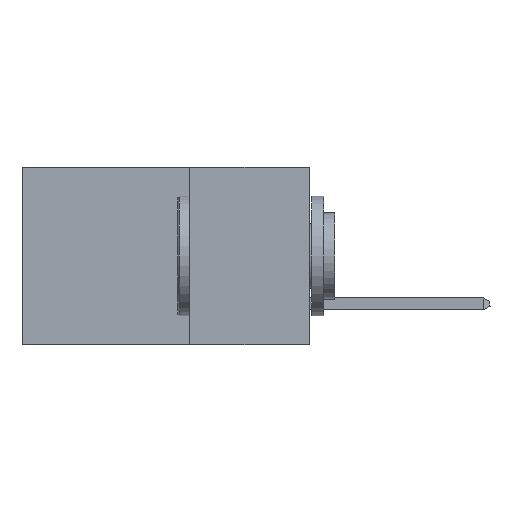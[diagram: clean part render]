
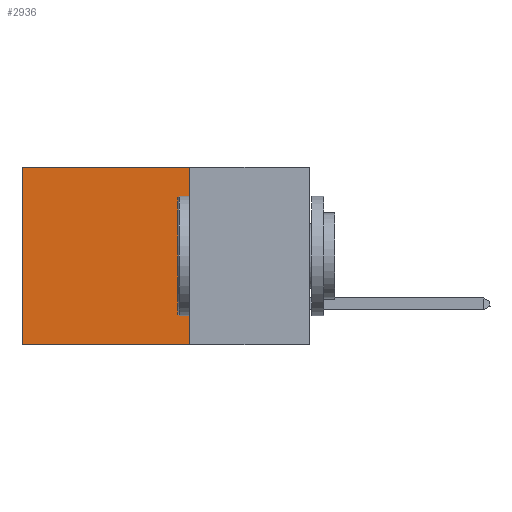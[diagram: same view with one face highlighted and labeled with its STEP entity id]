
A CAD part, left-side view. The second image highlights one B-rep face of the part: STEP entity #2936.
In plain terms, the highlighted planar face has unit normal (-1, 0, 0).
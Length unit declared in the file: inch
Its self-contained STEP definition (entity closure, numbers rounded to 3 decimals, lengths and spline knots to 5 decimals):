
#275 = VERTEX_POINT ( 'NONE', #2240 ) ;
#648 = VECTOR ( 'NONE', #9031, 39.37008 ) ;
#945 = EDGE_CURVE ( 'NONE', #275, #1674, #11428, .T. ) ;
#1343 = ORIENTED_EDGE ( 'NONE', *, *, #3459, .T. ) ;
#1512 = CARTESIAN_POINT ( 'NONE',  ( 0.2875, 0.6, 0. ) ) ;
#1674 = VERTEX_POINT ( 'NONE', #7368 ) ;
#2240 = CARTESIAN_POINT ( 'NONE',  ( 0.2875, 0.25, 0. ) ) ;
#2512 = DIRECTION ( 'NONE',  ( 1., 0., 0. ) ) ;
#2647 = AXIS2_PLACEMENT_3D ( 'NONE', #8001, #2512, #8926 ) ;
#2830 = CARTESIAN_POINT ( 'NONE',  ( 0.2875, 0.6, 0. ) ) ;
#2936 = ADVANCED_FACE ( 'NONE', ( #5419 ), #4305, .F. ) ;
#3459 = EDGE_CURVE ( 'NONE', #9494, #3676, #11874, .T. ) ;
#3676 = VERTEX_POINT ( 'NONE', #9169 ) ;
#3939 = DIRECTION ( 'NONE',  ( 0., 1., 0. ) ) ;
#4305 = PLANE ( 'NONE',  #2647 ) ;
#4887 = CARTESIAN_POINT ( 'NONE',  ( 0.2875, 0.25, 0. ) ) ;
#5370 = DIRECTION ( 'NONE',  ( 0., 0., -1. ) ) ;
#5419 = FACE_OUTER_BOUND ( 'NONE', #9442, .T. ) ;
#6614 = LINE ( 'NONE', #11047, #8190 ) ;
#7368 = CARTESIAN_POINT ( 'NONE',  ( 0.2875, 0.25, -0.37 ) ) ;
#8001 = CARTESIAN_POINT ( 'NONE',  ( 0.2875, 0.25, 0. ) ) ;
#8190 = VECTOR ( 'NONE', #3939, 39.37008 ) ;
#8768 = ORIENTED_EDGE ( 'NONE', *, *, #945, .F. ) ;
#8926 = DIRECTION ( 'NONE',  ( 0., 0., -1. ) ) ;
#9031 = DIRECTION ( 'NONE',  ( 0., 1., 0. ) ) ;
#9169 = CARTESIAN_POINT ( 'NONE',  ( 0.2875, 0.6, -0.37 ) ) ;
#9361 = ORIENTED_EDGE ( 'NONE', *, *, #11717, .T. ) ;
#9423 = VECTOR ( 'NONE', #5370, 39.37008 ) ;
#9435 = EDGE_CURVE ( 'NONE', #1674, #3676, #6614, .T. ) ;
#9442 = EDGE_LOOP ( 'NONE', ( #1343, #9548, #8768, #9361 ) ) ;
#9494 = VERTEX_POINT ( 'NONE', #2830 ) ;
#9548 = ORIENTED_EDGE ( 'NONE', *, *, #9435, .F. ) ;
#9983 = LINE ( 'NONE', #10937, #648 ) ;
#10937 = CARTESIAN_POINT ( 'NONE',  ( 0.2875, 0.25, 0. ) ) ;
#11047 = CARTESIAN_POINT ( 'NONE',  ( 0.2875, 0.25, -0.37 ) ) ;
#11236 = DIRECTION ( 'NONE',  ( 0., 0., -1. ) ) ;
#11428 = LINE ( 'NONE', #4887, #11455 ) ;
#11455 = VECTOR ( 'NONE', #11236, 39.37008 ) ;
#11717 = EDGE_CURVE ( 'NONE', #275, #9494, #9983, .T. ) ;
#11874 = LINE ( 'NONE', #1512, #9423 ) ;
